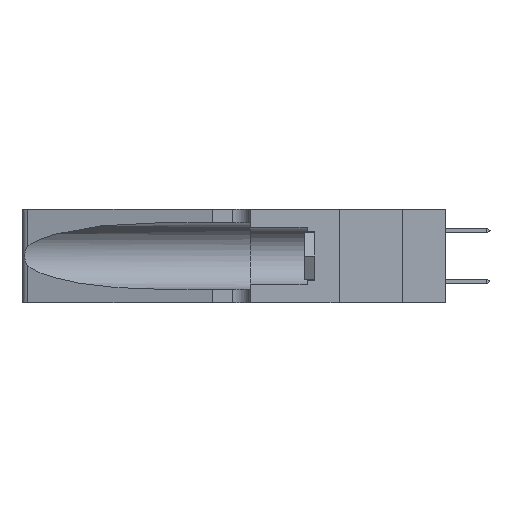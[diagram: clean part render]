
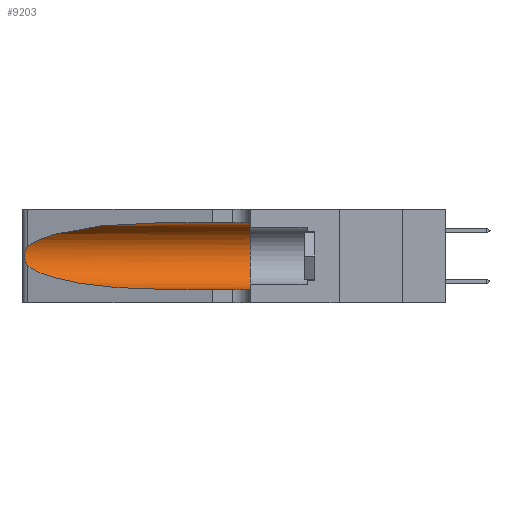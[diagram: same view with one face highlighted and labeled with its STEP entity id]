
A CAD part, left-side view. The second image highlights one B-rep face of the part: STEP entity #9203.
In plain terms, the highlighted cylindrical face has radius 3.308 mm (diameter 6.617 mm), a partial arc.
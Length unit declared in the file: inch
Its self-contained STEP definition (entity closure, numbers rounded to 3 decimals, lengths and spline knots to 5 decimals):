
#346 = CIRCLE ( 'NONE', #22876, 0.13025 ) ;
#394 = CARTESIAN_POINT ( 'NONE',  ( 0.1305, 0.35, 0.05475 ) ) ;
#844 = VERTEX_POINT ( 'NONE', #7817 ) ;
#1265 = VERTEX_POINT ( 'NONE', #13303 ) ;
#1733 = CARTESIAN_POINT ( 'NONE',  ( 0.26018, 1.23835, 0.19895 ) ) ;
#3237 = CARTESIAN_POINT ( 'NONE',  ( 0.2373, 1.15595, 0.08982 ) ) ;
#3846 = CARTESIAN_POINT ( 'NONE',  ( 0.26075, 1.23896, 0.178 ) ) ;
#4434 = CARTESIAN_POINT ( 'NONE',  ( 0.1305, 1.61858, 0.185 ) ) ;
#5279 = CARTESIAN_POINT ( 'NONE',  ( 0.2373, 1.15595, 0.28018 ) ) ;
#5443 = CARTESIAN_POINT ( 'NONE',  ( 0.1305, 0.72297, 0.05475 ) ) ;
#5932 = CARTESIAN_POINT ( 'NONE',  ( 0.25856, 1.23593, 0.16098 ) ) ;
#5963 = LINE ( 'NONE', #10304, #16979 ) ;
#5996 = CARTESIAN_POINT ( 'NONE',  ( 0.1305, 0.35, 0.185 ) ) ;
#6054 = CYLINDRICAL_SURFACE ( 'NONE', #11864, 0.13025 ) ;
#6893 = EDGE_CURVE ( 'NONE', #16667, #14485, #19785, .T. ) ;
#7152 = LINE ( 'NONE', #13410, #23047 ) ;
#7817 = CARTESIAN_POINT ( 'NONE',  ( 0.1305, 0.35, 0.31525 ) ) ;
#7919 = CARTESIAN_POINT ( 'NONE',  ( 0.25487, 1.22718, 0.22369 ) ) ;
#8011 = CARTESIAN_POINT ( 'NONE',  ( 0.25639, 1.23186, 0.15144 ) ) ;
#8074 = DIRECTION ( 'NONE',  ( 0., 0., 1. ) ) ;
#8606 = DIRECTION ( 'NONE',  ( 0., 0., -1. ) ) ;
#9139 = EDGE_LOOP ( 'NONE', ( #25610, #20010, #21951, #24817, #13394, #15987 ) ) ;
#9203 = ADVANCED_FACE ( 'NONE', ( #17066 ), #6054, .F. ) ;
#9436 = CARTESIAN_POINT ( 'NONE',  ( 0.1305, 0.72297, 0.31525 ) ) ;
#10093 = CARTESIAN_POINT ( 'NONE',  ( 0.25487, 1.22718, 0.14631 ) ) ;
#10304 = CARTESIAN_POINT ( 'NONE',  ( 0.1305, 1.61858, 0.05475 ) ) ;
#11864 = AXIS2_PLACEMENT_3D ( 'NONE', #4434, #25118, #8606 ) ;
#12082 = CARTESIAN_POINT ( 'NONE',  ( 0.25639, 1.23184, 0.21858 ) ) ;
#12290 = EDGE_CURVE ( 'NONE', #16667, #844, #7152, .T. ) ;
#12371 = DIRECTION ( 'NONE',  ( 0., -1., 0. ) ) ;
#12949 = B_SPLINE_CURVE_WITH_KNOTS ( 'NONE', 3,
 ( #7919, #16135, #12082, #26586, #14150, #1733, #16229, #3846, #18337, #5932, #20429, #8011, #22493, #10093 ),
 .UNSPECIFIED., .F., .F.,
 ( 4, 2, 2, 2, 2, 2, 4 ),
 ( 0., 0.00027, 0.00053, 0.00107, 0.0016, 0.00187, 0.00214 ),
 .UNSPECIFIED. ) ;
#13303 = CARTESIAN_POINT ( 'NONE',  ( 0.25487, 1.22718, 0.14631 ) ) ;
#13394 = ORIENTED_EDGE ( 'NONE', *, *, #18990, .F. ) ;
#13410 = CARTESIAN_POINT ( 'NONE',  ( 0.1305, 1.61858, 0.31525 ) ) ;
#14150 = CARTESIAN_POINT ( 'NONE',  ( 0.25854, 1.2359, 0.20912 ) ) ;
#14264 = CARTESIAN_POINT ( 'NONE',  ( 0.25487, 1.22718, 0.22369 ) ) ;
#14328 = EDGE_CURVE ( 'NONE', #1265, #26469, #22582, .T. ) ;
#14485 = VERTEX_POINT ( 'NONE', #14264 ) ;
#15565 = CARTESIAN_POINT ( 'NONE',  ( 0.18966, 0.96281, 0.31525 ) ) ;
#15623 = CARTESIAN_POINT ( 'NONE',  ( 0.25487, 1.22718, 0.14631 ) ) ;
#15987 = ORIENTED_EDGE ( 'NONE', *, *, #12290, .F. ) ;
#16135 = CARTESIAN_POINT ( 'NONE',  ( 0.25555, 1.22994, 0.2215 ) ) ;
#16229 = CARTESIAN_POINT ( 'NONE',  ( 0.26075, 1.23896, 0.19203 ) ) ;
#16667 = VERTEX_POINT ( 'NONE', #23113 ) ;
#16979 = VECTOR ( 'NONE', #12371, 39.37008 ) ;
#17066 = FACE_OUTER_BOUND ( 'NONE', #9139, .T. ) ;
#17828 = CARTESIAN_POINT ( 'NONE',  ( 0.18966, 0.96281, 0.05475 ) ) ;
#17848 = EDGE_CURVE ( 'NONE', #26469, #23097, #5963, .T. ) ;
#18337 = CARTESIAN_POINT ( 'NONE',  ( 0.26017, 1.23833, 0.17102 ) ) ;
#18371 = EDGE_CURVE ( 'NONE', #14485, #1265, #12949, .T. ) ;
#18990 = EDGE_CURVE ( 'NONE', #844, #23097, #346, .T. ) ;
#19323 = CARTESIAN_POINT ( 'NONE',  ( 0.1305, 0.72297, 0.05475 ) ) ;
#19785 =( BOUNDED_CURVE ( )  B_SPLINE_CURVE ( 3, ( #9436, #15565, #5279, #23951 ),
 .UNSPECIFIED., .F., .F. ) 
 B_SPLINE_CURVE_WITH_KNOTS ( ( 4, 4 ),
 ( 1.5708, 2.84003 ),
 .UNSPECIFIED. ) 
 CURVE ( )  GEOMETRIC_REPRESENTATION_ITEM ( )  RATIONAL_B_SPLINE_CURVE ( ( 1., 0.87, 0.87, 1. ) ) 
 REPRESENTATION_ITEM ( '' )  );
#20010 = ORIENTED_EDGE ( 'NONE', *, *, #18371, .T. ) ;
#20429 = CARTESIAN_POINT ( 'NONE',  ( 0.25789, 1.23486, 0.15765 ) ) ;
#20483 = DIRECTION ( 'NONE',  ( 0., 1., 0. ) ) ;
#21951 = ORIENTED_EDGE ( 'NONE', *, *, #14328, .T. ) ;
#22493 = CARTESIAN_POINT ( 'NONE',  ( 0.25555, 1.22993, 0.14849 ) ) ;
#22582 =( BOUNDED_CURVE ( )  B_SPLINE_CURVE ( 3, ( #15623, #3237, #17828, #5443 ),
 .UNSPECIFIED., .F., .F. ) 
 B_SPLINE_CURVE_WITH_KNOTS ( ( 4, 4 ),
 ( 3.44316, 4.71239 ),
 .UNSPECIFIED. ) 
 CURVE ( )  GEOMETRIC_REPRESENTATION_ITEM ( )  RATIONAL_B_SPLINE_CURVE ( ( 1., 0.87, 0.87, 1. ) ) 
 REPRESENTATION_ITEM ( '' )  );
#22876 = AXIS2_PLACEMENT_3D ( 'NONE', #5996, #20483, #8074 ) ;
#23047 = VECTOR ( 'NONE', #23782, 39.37008 ) ;
#23097 = VERTEX_POINT ( 'NONE', #394 ) ;
#23113 = CARTESIAN_POINT ( 'NONE',  ( 0.1305, 0.72297, 0.31525 ) ) ;
#23782 = DIRECTION ( 'NONE',  ( 0., -1., 0. ) ) ;
#23951 = CARTESIAN_POINT ( 'NONE',  ( 0.25487, 1.22718, 0.22369 ) ) ;
#24817 = ORIENTED_EDGE ( 'NONE', *, *, #17848, .T. ) ;
#25118 = DIRECTION ( 'NONE',  ( 0., -1., 0. ) ) ;
#25610 = ORIENTED_EDGE ( 'NONE', *, *, #6893, .T. ) ;
#26469 = VERTEX_POINT ( 'NONE', #19323 ) ;
#26586 = CARTESIAN_POINT ( 'NONE',  ( 0.25787, 1.23484, 0.2124 ) ) ;
